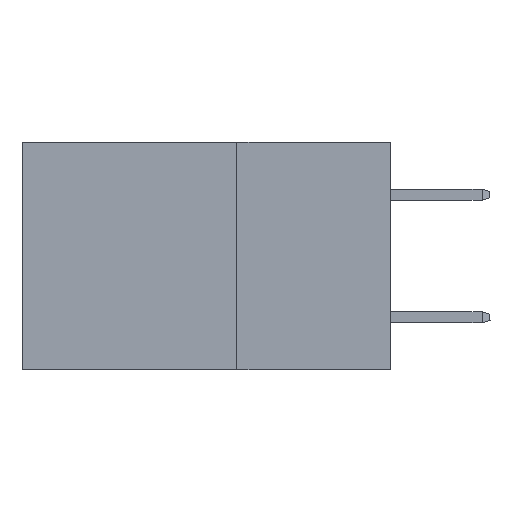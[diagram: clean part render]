
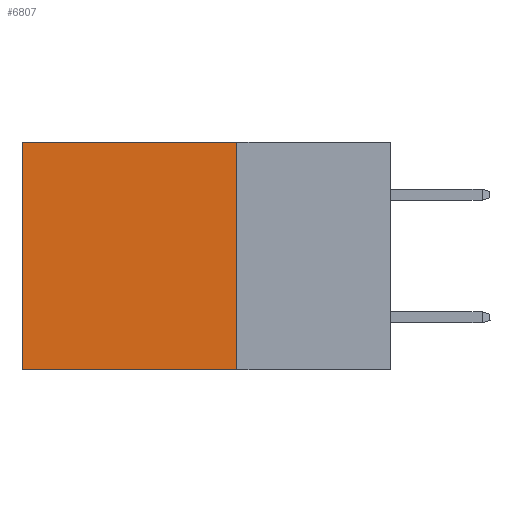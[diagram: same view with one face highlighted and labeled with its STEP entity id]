
A CAD part, left-side view. The second image highlights one B-rep face of the part: STEP entity #6807.
In plain terms, the highlighted planar face has unit normal (-1, 0, 0).
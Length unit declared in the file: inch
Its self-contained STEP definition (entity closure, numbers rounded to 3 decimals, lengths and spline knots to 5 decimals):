
#878 = CARTESIAN_POINT ( 'NONE',  ( 0.2875, 0.6, 0. ) ) ;
#951 = CARTESIAN_POINT ( 'NONE',  ( 0.2875, 0.6, 0. ) ) ;
#1144 = CARTESIAN_POINT ( 'NONE',  ( 0.2875, 0.25, 0. ) ) ;
#3011 = ORIENTED_EDGE ( 'NONE', *, *, #34022, .F. ) ;
#3089 = DIRECTION ( 'NONE',  ( 0., 0., -1. ) ) ;
#3307 = VECTOR ( 'NONE', #10440, 39.37008 ) ;
#5951 = CARTESIAN_POINT ( 'NONE',  ( 0.2875, 0.25, 0. ) ) ;
#6807 = ADVANCED_FACE ( 'NONE', ( #15848 ), #31060, .F. ) ;
#8315 = VERTEX_POINT ( 'NONE', #23824 ) ;
#9051 = VECTOR ( 'NONE', #39429, 39.37008 ) ;
#10440 = DIRECTION ( 'NONE',  ( 0., 0., -1. ) ) ;
#11449 = VERTEX_POINT ( 'NONE', #878 ) ;
#11544 = CARTESIAN_POINT ( 'NONE',  ( 0.2875, 0.25, 0. ) ) ;
#12150 = EDGE_CURVE ( 'NONE', #25064, #11449, #12540, .T. ) ;
#12397 = EDGE_CURVE ( 'NONE', #27440, #8315, #12944, .T. ) ;
#12540 = LINE ( 'NONE', #5951, #30702 ) ;
#12641 = ORIENTED_EDGE ( 'NONE', *, *, #12397, .F. ) ;
#12944 = LINE ( 'NONE', #32859, #9051 ) ;
#14477 = ORIENTED_EDGE ( 'NONE', *, *, #12150, .T. ) ;
#14817 = DIRECTION ( 'NONE',  ( 0., 0., -1. ) ) ;
#15454 = VECTOR ( 'NONE', #14817, 39.37008 ) ;
#15750 = EDGE_CURVE ( 'NONE', #11449, #8315, #25843, .T. ) ;
#15827 = DIRECTION ( 'NONE',  ( 0., 1., 0. ) ) ;
#15848 = FACE_OUTER_BOUND ( 'NONE', #22071, .T. ) ;
#17161 = CARTESIAN_POINT ( 'NONE',  ( 0.2875, 0.25, -0.37 ) ) ;
#18737 = CARTESIAN_POINT ( 'NONE',  ( 0.2875, 0.25, 0. ) ) ;
#22071 = EDGE_LOOP ( 'NONE', ( #27065, #12641, #3011, #14477 ) ) ;
#23824 = CARTESIAN_POINT ( 'NONE',  ( 0.2875, 0.6, -0.37 ) ) ;
#25064 = VERTEX_POINT ( 'NONE', #1144 ) ;
#25843 = LINE ( 'NONE', #951, #3307 ) ;
#27065 = ORIENTED_EDGE ( 'NONE', *, *, #15750, .T. ) ;
#27440 = VERTEX_POINT ( 'NONE', #17161 ) ;
#27873 = AXIS2_PLACEMENT_3D ( 'NONE', #18737, #31268, #3089 ) ;
#30702 = VECTOR ( 'NONE', #15827, 39.37008 ) ;
#31057 = LINE ( 'NONE', #11544, #15454 ) ;
#31060 = PLANE ( 'NONE',  #27873 ) ;
#31268 = DIRECTION ( 'NONE',  ( 1., 0., 0. ) ) ;
#32859 = CARTESIAN_POINT ( 'NONE',  ( 0.2875, 0.25, -0.37 ) ) ;
#34022 = EDGE_CURVE ( 'NONE', #25064, #27440, #31057, .T. ) ;
#39429 = DIRECTION ( 'NONE',  ( 0., 1., 0. ) ) ;
